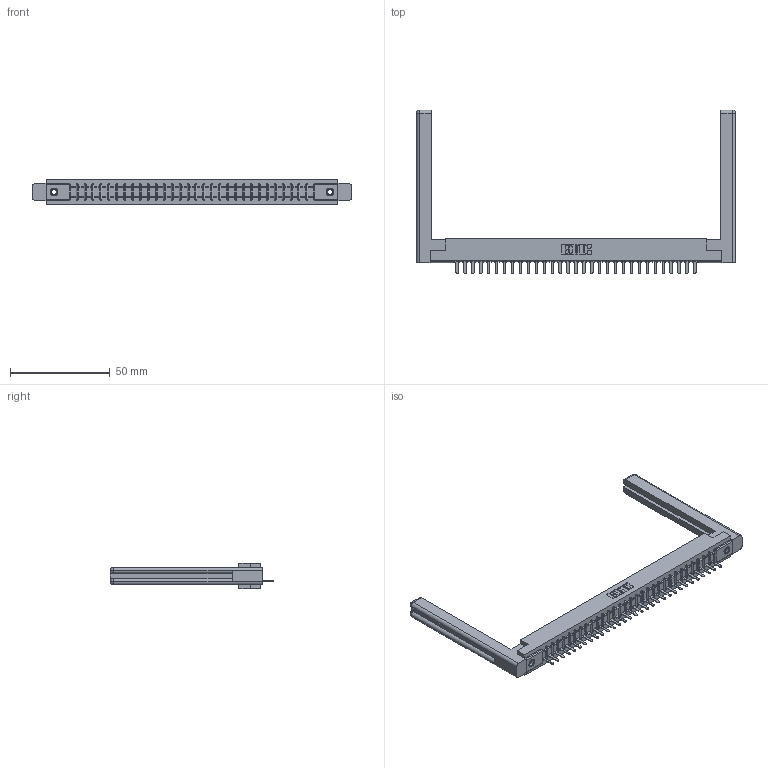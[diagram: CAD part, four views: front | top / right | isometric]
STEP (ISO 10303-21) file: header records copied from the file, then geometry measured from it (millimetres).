
FILE_DESCRIPTION (( 'STEP AP203' ), '1' );
FILE_NAME ('357-031-521-158.STEP', '2019-09-17T03:39:51', ( '' ), ( '' ), 'SwSTEP 2.0', 'SolidWorks 2016', '' );
FILE_SCHEMA (( 'CONFIG_CONTROL_DESIGN' ));
Length unit declared in the file: inch
Products named in the file (5): 307-220-058; 307 Part_.156 Dia Mounting Holes; 307-290-002_521; 357-031-521-158; 345-250-001_345-250-001-102
Assembly tree (36 placements, depth 2):
  357-031-521-158
    307 Part_.156 Dia Mounting Holes
    307-290-002_521  x31
    307-220-058  x2
    345-250-001_345-250-001-102  x2
Bounding box: 159.46 x 81.74 x 12.7 mm (x, y, z)
Volume: 24104.4 mm3; surface area: 25951.4 mm2
Topology: 36 solids, 36 shells, 2586 faces, 7869 edges, 5146 vertices
Faces by surface type: plane 1549, cylinder 949, sphere 64, torus 12, cone 12
Entity records: 31283 total; most frequent: CARTESIAN_POINT 5283, ORIENTED_EDGE 5212, DIRECTION 5098, EDGE_CURVE 2606, VECTOR 1988, LINE 1988, VERTEX_POINT 1686, AXIS2_PLACEMENT_3D 1555
